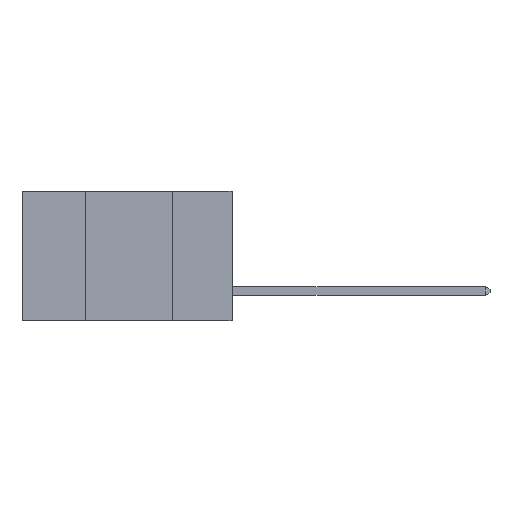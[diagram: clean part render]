
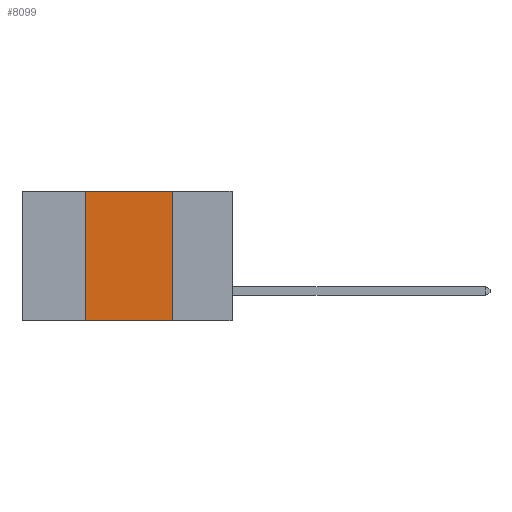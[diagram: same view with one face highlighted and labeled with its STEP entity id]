
A CAD part, left-side view. The second image highlights one B-rep face of the part: STEP entity #8099.
In plain terms, the highlighted planar face has unit normal (-1, 0, 0).
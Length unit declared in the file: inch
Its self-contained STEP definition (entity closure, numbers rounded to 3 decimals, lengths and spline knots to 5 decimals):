
#183 = LINE ( 'NONE', #16049, #18252 ) ;
#334 = VERTEX_POINT ( 'NONE', #19553 ) ;
#1134 = EDGE_CURVE ( 'NONE', #11139, #6348, #21429, .T. ) ;
#1368 = VERTEX_POINT ( 'NONE', #2310 ) ;
#1591 = PLANE ( 'NONE',  #11656 ) ;
#1610 = ORIENTED_EDGE ( 'NONE', *, *, #2799, .F. ) ;
#2310 = CARTESIAN_POINT ( 'NONE',  ( 0., 0.17, 0. ) ) ;
#2615 = CARTESIAN_POINT ( 'NONE',  ( 0., 0.17, -0.37 ) ) ;
#2799 = EDGE_CURVE ( 'NONE', #334, #1368, #183, .T. ) ;
#3982 = CARTESIAN_POINT ( 'NONE',  ( 0., 0.42, 0. ) ) ;
#4051 = ORIENTED_EDGE ( 'NONE', *, *, #22471, .F. ) ;
#4239 = ORIENTED_EDGE ( 'NONE', *, *, #8199, .F. ) ;
#4866 = VECTOR ( 'NONE', #21180, 39.37008 ) ;
#5168 = CARTESIAN_POINT ( 'NONE',  ( 0., 0.6, 0. ) ) ;
#5760 = DIRECTION ( 'NONE',  ( 0., 0., 1. ) ) ;
#6348 = VERTEX_POINT ( 'NONE', #2615 ) ;
#6901 = DIRECTION ( 'NONE',  ( 1., 0., 0. ) ) ;
#7401 = DIRECTION ( 'NONE',  ( 0., -1., 0. ) ) ;
#8099 = ADVANCED_FACE ( 'NONE', ( #10080 ), #1591, .F. ) ;
#8199 = EDGE_CURVE ( 'NONE', #1368, #6348, #12876, .T. ) ;
#9175 = ORIENTED_EDGE ( 'NONE', *, *, #1134, .T. ) ;
#9711 = DIRECTION ( 'NONE',  ( 0., -1., 0. ) ) ;
#10080 = FACE_OUTER_BOUND ( 'NONE', #20473, .T. ) ;
#10855 = CARTESIAN_POINT ( 'NONE',  ( 0., 0.17, 0. ) ) ;
#11139 = VERTEX_POINT ( 'NONE', #17431 ) ;
#11656 = AXIS2_PLACEMENT_3D ( 'NONE', #5168, #6901, #19053 ) ;
#12120 = LINE ( 'NONE', #3982, #20766 ) ;
#12876 = LINE ( 'NONE', #10855, #4866 ) ;
#14500 = CARTESIAN_POINT ( 'NONE',  ( 0., 0.6, -0.37 ) ) ;
#16049 = CARTESIAN_POINT ( 'NONE',  ( 0., 0.6, 0. ) ) ;
#16907 = VECTOR ( 'NONE', #9711, 39.37008 ) ;
#17431 = CARTESIAN_POINT ( 'NONE',  ( 0., 0.42, -0.37 ) ) ;
#18252 = VECTOR ( 'NONE', #7401, 39.37008 ) ;
#19053 = DIRECTION ( 'NONE',  ( 0., 0., -1. ) ) ;
#19553 = CARTESIAN_POINT ( 'NONE',  ( 0., 0.42, 0. ) ) ;
#20473 = EDGE_LOOP ( 'NONE', ( #4239, #1610, #4051, #9175 ) ) ;
#20766 = VECTOR ( 'NONE', #5760, 39.37008 ) ;
#21180 = DIRECTION ( 'NONE',  ( 0., 0., -1. ) ) ;
#21429 = LINE ( 'NONE', #14500, #16907 ) ;
#22471 = EDGE_CURVE ( 'NONE', #11139, #334, #12120, .T. ) ;
